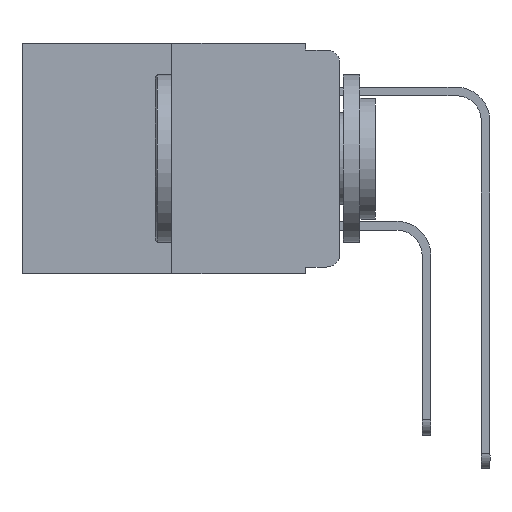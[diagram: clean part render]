
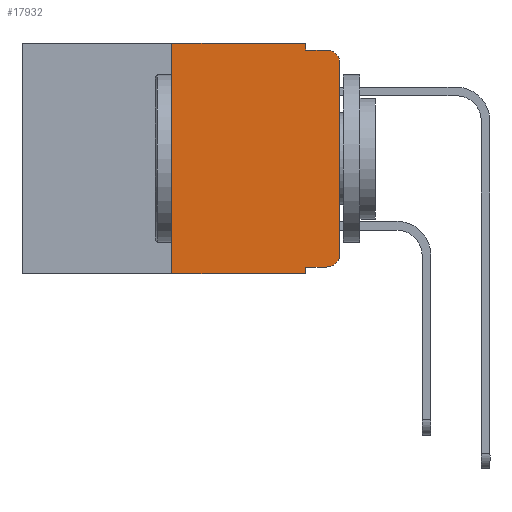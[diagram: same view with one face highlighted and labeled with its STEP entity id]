
A CAD part, left-side view. The second image highlights one B-rep face of the part: STEP entity #17932.
In plain terms, the highlighted planar face has unit normal (-1, 0, 0).
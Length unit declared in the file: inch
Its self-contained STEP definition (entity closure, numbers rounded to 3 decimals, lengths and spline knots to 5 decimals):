
#49 = CARTESIAN_POINT ( 'NONE',  ( 0., 0.051, -0.333 ) ) ;
#476 = DIRECTION ( 'NONE',  ( -1., 0., 0. ) ) ;
#664 = CARTESIAN_POINT ( 'NONE',  ( 0., 0.25, -0.343 ) ) ;
#687 = DIRECTION ( 'NONE',  ( 0., 0., -1. ) ) ;
#1080 = CIRCLE ( 'NONE', #9722, 0.02 ) ;
#1108 = VECTOR ( 'NONE', #14833, 39.37008 ) ;
#1460 = LINE ( 'NONE', #8010, #17129 ) ;
#1564 = DIRECTION ( 'NONE',  ( -1., 0., 0. ) ) ;
#1616 = DIRECTION ( 'NONE',  ( 0., 0., -1. ) ) ;
#1640 = EDGE_CURVE ( 'NONE', #10778, #7455, #4079, .T. ) ;
#1651 = ORIENTED_EDGE ( 'NONE', *, *, #1776, .F. ) ;
#1776 = EDGE_CURVE ( 'NONE', #19920, #2839, #1460, .T. ) ;
#2202 = VECTOR ( 'NONE', #1616, 39.37008 ) ;
#2320 = EDGE_LOOP ( 'NONE', ( #7724, #7135, #7879, #1651, #13615, #16317, #5754, #9568, #6860, #11178 ) ) ;
#2330 = CARTESIAN_POINT ( 'NONE',  ( 0., 0.051, -0.343 ) ) ;
#2432 = DIRECTION ( 'NONE',  ( 1., 0., 0. ) ) ;
#2739 = CIRCLE ( 'NONE', #12801, 0.02 ) ;
#2839 = VERTEX_POINT ( 'NONE', #11156 ) ;
#2872 = VECTOR ( 'NONE', #14818, 39.37008 ) ;
#3322 = VERTEX_POINT ( 'NONE', #5740 ) ;
#4079 = LINE ( 'NONE', #18018, #14978 ) ;
#4089 = CARTESIAN_POINT ( 'NONE',  ( 0., 0.051, 0. ) ) ;
#4308 = EDGE_CURVE ( 'NONE', #11063, #3322, #7979, .T. ) ;
#4500 = DIRECTION ( 'NONE',  ( 0., -1., 0. ) ) ;
#4800 = CARTESIAN_POINT ( 'NONE',  ( 0., 0.051, -0.01 ) ) ;
#4945 = DIRECTION ( 'NONE',  ( 0., 0., -1. ) ) ;
#5143 = EDGE_CURVE ( 'NONE', #3322, #15851, #2739, .T. ) ;
#5740 = CARTESIAN_POINT ( 'NONE',  ( 0., 0., -0.03 ) ) ;
#5754 = ORIENTED_EDGE ( 'NONE', *, *, #9668, .T. ) ;
#5832 = PLANE ( 'NONE',  #16584 ) ;
#6018 = EDGE_CURVE ( 'NONE', #8354, #17840, #6602, .T. ) ;
#6056 = CARTESIAN_POINT ( 'NONE',  ( 0., 0.02, -0.01 ) ) ;
#6062 = CARTESIAN_POINT ( 'NONE',  ( 0., 0., 0. ) ) ;
#6195 = LINE ( 'NONE', #18969, #19406 ) ;
#6602 = LINE ( 'NONE', #8387, #2202 ) ;
#6860 = ORIENTED_EDGE ( 'NONE', *, *, #22268, .T. ) ;
#7135 = ORIENTED_EDGE ( 'NONE', *, *, #5143, .T. ) ;
#7455 = VERTEX_POINT ( 'NONE', #14226 ) ;
#7634 = FACE_OUTER_BOUND ( 'NONE', #2320, .T. ) ;
#7724 = ORIENTED_EDGE ( 'NONE', *, *, #4308, .T. ) ;
#7879 = ORIENTED_EDGE ( 'NONE', *, *, #12670, .F. ) ;
#7979 = LINE ( 'NONE', #6062, #1108 ) ;
#8010 = CARTESIAN_POINT ( 'NONE',  ( 0., 0.051, 0. ) ) ;
#8354 = VERTEX_POINT ( 'NONE', #49 ) ;
#8387 = CARTESIAN_POINT ( 'NONE',  ( 0., 0.051, 0. ) ) ;
#8749 = LINE ( 'NONE', #20683, #18879 ) ;
#9539 = DIRECTION ( 'NONE',  ( 0., 0., -1. ) ) ;
#9568 = ORIENTED_EDGE ( 'NONE', *, *, #6018, .F. ) ;
#9668 = EDGE_CURVE ( 'NONE', #10778, #17840, #6195, .T. ) ;
#9722 = AXIS2_PLACEMENT_3D ( 'NONE', #16112, #476, #687 ) ;
#10248 = DIRECTION ( 'NONE',  ( 0., -1., 0. ) ) ;
#10778 = VERTEX_POINT ( 'NONE', #664 ) ;
#10996 = CARTESIAN_POINT ( 'NONE',  ( 0., 0.473, 0. ) ) ;
#11063 = VERTEX_POINT ( 'NONE', #17531 ) ;
#11156 = CARTESIAN_POINT ( 'NONE',  ( 0., 0.051, -0.01 ) ) ;
#11178 = ORIENTED_EDGE ( 'NONE', *, *, #13445, .T. ) ;
#11806 = LINE ( 'NONE', #18800, #21689 ) ;
#12644 = CARTESIAN_POINT ( 'NONE',  ( 0., 0.02, -0.03 ) ) ;
#12670 = EDGE_CURVE ( 'NONE', #2839, #15851, #16732, .T. ) ;
#12801 = AXIS2_PLACEMENT_3D ( 'NONE', #12644, #1564, #4945 ) ;
#12838 = DIRECTION ( 'NONE',  ( 0., 0., 1. ) ) ;
#13445 = EDGE_CURVE ( 'NONE', #15881, #11063, #1080, .T. ) ;
#13615 = ORIENTED_EDGE ( 'NONE', *, *, #17110, .F. ) ;
#14226 = CARTESIAN_POINT ( 'NONE',  ( 0., 0.25, 0. ) ) ;
#14705 = CARTESIAN_POINT ( 'NONE',  ( 0., 0.02, -0.333 ) ) ;
#14818 = DIRECTION ( 'NONE',  ( 0., -1., 0. ) ) ;
#14833 = DIRECTION ( 'NONE',  ( 0., 0., 1. ) ) ;
#14978 = VECTOR ( 'NONE', #12838, 39.37008 ) ;
#15604 = DIRECTION ( 'NONE',  ( 0., -1., 0. ) ) ;
#15851 = VERTEX_POINT ( 'NONE', #6056 ) ;
#15881 = VERTEX_POINT ( 'NONE', #14705 ) ;
#16112 = CARTESIAN_POINT ( 'NONE',  ( 0., 0.02, -0.313 ) ) ;
#16317 = ORIENTED_EDGE ( 'NONE', *, *, #1640, .F. ) ;
#16584 = AXIS2_PLACEMENT_3D ( 'NONE', #10996, #2432, #9539 ) ;
#16732 = LINE ( 'NONE', #4800, #2872 ) ;
#17110 = EDGE_CURVE ( 'NONE', #7455, #19920, #11806, .T. ) ;
#17129 = VECTOR ( 'NONE', #21968, 39.37008 ) ;
#17531 = CARTESIAN_POINT ( 'NONE',  ( 0., 0., -0.313 ) ) ;
#17840 = VERTEX_POINT ( 'NONE', #2330 ) ;
#17932 = ADVANCED_FACE ( 'NONE', ( #7634 ), #5832, .F. ) ;
#18018 = CARTESIAN_POINT ( 'NONE',  ( 0., 0.25, 0. ) ) ;
#18800 = CARTESIAN_POINT ( 'NONE',  ( 0., 0.473, 0. ) ) ;
#18879 = VECTOR ( 'NONE', #15604, 39.37008 ) ;
#18969 = CARTESIAN_POINT ( 'NONE',  ( 0., 0.473, -0.343 ) ) ;
#19406 = VECTOR ( 'NONE', #4500, 39.37008 ) ;
#19920 = VERTEX_POINT ( 'NONE', #4089 ) ;
#20683 = CARTESIAN_POINT ( 'NONE',  ( 0., 0.051, -0.333 ) ) ;
#21689 = VECTOR ( 'NONE', #10248, 39.37008 ) ;
#21968 = DIRECTION ( 'NONE',  ( 0., 0., -1. ) ) ;
#22268 = EDGE_CURVE ( 'NONE', #8354, #15881, #8749, .T. ) ;
